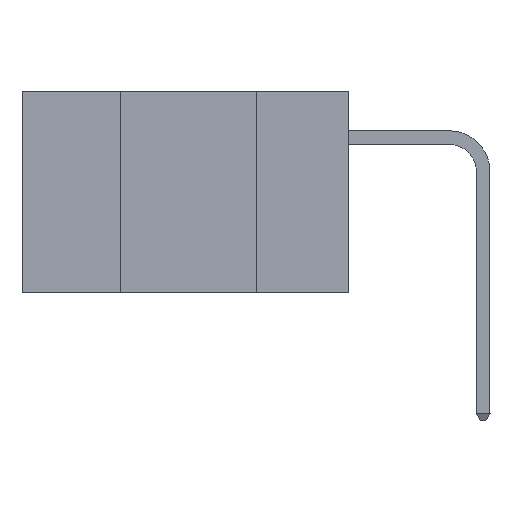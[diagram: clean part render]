
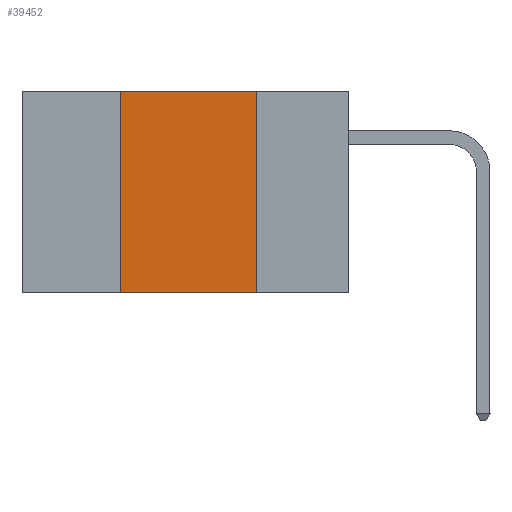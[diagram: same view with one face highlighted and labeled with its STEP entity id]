
A CAD part, left-side view. The second image highlights one B-rep face of the part: STEP entity #39452.
In plain terms, the highlighted planar face has unit normal (-1, 0, 0).
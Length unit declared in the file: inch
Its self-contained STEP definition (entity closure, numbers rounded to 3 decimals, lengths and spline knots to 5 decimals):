
#314 = LINE ( 'NONE', #5842, #7161 ) ;
#1066 = EDGE_LOOP ( 'NONE', ( #16823, #4166, #27223, #36377 ) ) ;
#2864 = CARTESIAN_POINT ( 'NONE',  ( 0., 0.42, 0. ) ) ;
#4166 = ORIENTED_EDGE ( 'NONE', *, *, #18173, .F. ) ;
#5842 = CARTESIAN_POINT ( 'NONE',  ( 0., 0.6, -0.37 ) ) ;
#7161 = VECTOR ( 'NONE', #25186, 39.37008 ) ;
#9970 = CARTESIAN_POINT ( 'NONE',  ( 0., 0.42, 0. ) ) ;
#12785 = FACE_OUTER_BOUND ( 'NONE', #1066, .T. ) ;
#16823 = ORIENTED_EDGE ( 'NONE', *, *, #35307, .F. ) ;
#17382 = CARTESIAN_POINT ( 'NONE',  ( 0., 0.17, 0. ) ) ;
#17711 = CARTESIAN_POINT ( 'NONE',  ( 0., 0.42, -0.37 ) ) ;
#18173 = EDGE_CURVE ( 'NONE', #27016, #29119, #35449, .T. ) ;
#18295 = VERTEX_POINT ( 'NONE', #38231 ) ;
#19622 = LINE ( 'NONE', #17382, #29990 ) ;
#21014 = AXIS2_PLACEMENT_3D ( 'NONE', #25000, #37434, #25399 ) ;
#21715 = CARTESIAN_POINT ( 'NONE',  ( 0., 0.17, 0. ) ) ;
#22122 = EDGE_CURVE ( 'NONE', #24598, #27016, #30806, .T. ) ;
#23315 = VECTOR ( 'NONE', #32201, 39.37008 ) ;
#24598 = VERTEX_POINT ( 'NONE', #17711 ) ;
#25000 = CARTESIAN_POINT ( 'NONE',  ( 0., 0.6, 0. ) ) ;
#25186 = DIRECTION ( 'NONE',  ( 0., -1., 0. ) ) ;
#25399 = DIRECTION ( 'NONE',  ( 0., 0., -1. ) ) ;
#27016 = VERTEX_POINT ( 'NONE', #9970 ) ;
#27223 = ORIENTED_EDGE ( 'NONE', *, *, #22122, .F. ) ;
#27728 = DIRECTION ( 'NONE',  ( 0., 0., 1. ) ) ;
#29119 = VERTEX_POINT ( 'NONE', #21715 ) ;
#29329 = CARTESIAN_POINT ( 'NONE',  ( 0., 0.6, 0. ) ) ;
#29990 = VECTOR ( 'NONE', #39919, 39.37008 ) ;
#30806 = LINE ( 'NONE', #2864, #32553 ) ;
#32201 = DIRECTION ( 'NONE',  ( 0., -1., 0. ) ) ;
#32553 = VECTOR ( 'NONE', #27728, 39.37008 ) ;
#34729 = EDGE_CURVE ( 'NONE', #24598, #18295, #314, .T. ) ;
#35307 = EDGE_CURVE ( 'NONE', #29119, #18295, #19622, .T. ) ;
#35449 = LINE ( 'NONE', #29329, #23315 ) ;
#36377 = ORIENTED_EDGE ( 'NONE', *, *, #34729, .T. ) ;
#37434 = DIRECTION ( 'NONE',  ( 1., 0., 0. ) ) ;
#38024 = PLANE ( 'NONE',  #21014 ) ;
#38231 = CARTESIAN_POINT ( 'NONE',  ( 0., 0.17, -0.37 ) ) ;
#39452 = ADVANCED_FACE ( 'NONE', ( #12785 ), #38024, .F. ) ;
#39919 = DIRECTION ( 'NONE',  ( 0., 0., -1. ) ) ;
